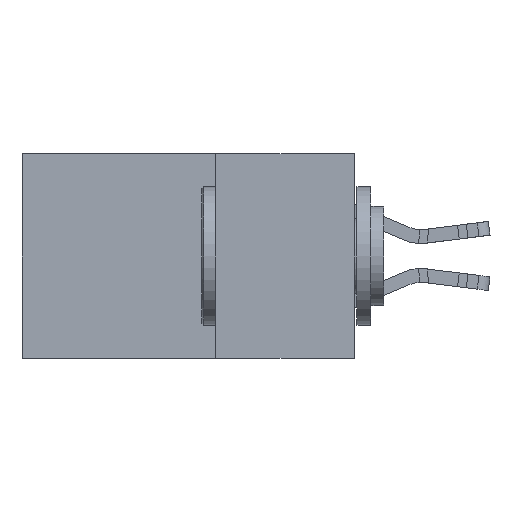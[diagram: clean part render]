
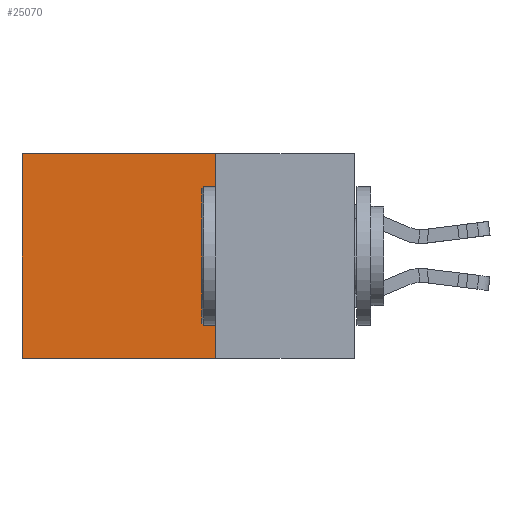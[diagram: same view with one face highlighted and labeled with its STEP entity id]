
A CAD part, left-side view. The second image highlights one B-rep face of the part: STEP entity #25070.
In plain terms, the highlighted planar face has unit normal (-1, 0, 0).
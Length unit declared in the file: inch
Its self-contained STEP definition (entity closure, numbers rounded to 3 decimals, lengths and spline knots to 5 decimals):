
#2036 = LINE ( 'NONE', #15305, #8247 ) ;
#2154 = VERTEX_POINT ( 'NONE', #5412 ) ;
#3725 = ORIENTED_EDGE ( 'NONE', *, *, #26143, .F. ) ;
#4687 = CARTESIAN_POINT ( 'NONE',  ( 0.2615, 0.25, 0. ) ) ;
#5412 = CARTESIAN_POINT ( 'NONE',  ( 0.2615, 0.6, 0. ) ) ;
#5791 = DIRECTION ( 'NONE',  ( 0., 1., 0. ) ) ;
#7809 = VECTOR ( 'NONE', #26336, 39.37008 ) ;
#8247 = VECTOR ( 'NONE', #10985, 39.37008 ) ;
#9611 = LINE ( 'NONE', #22758, #19324 ) ;
#10749 = VERTEX_POINT ( 'NONE', #24547 ) ;
#10985 = DIRECTION ( 'NONE',  ( 0., 0., -1. ) ) ;
#11311 = CARTESIAN_POINT ( 'NONE',  ( 0.2615, 0.25, -0.37 ) ) ;
#11790 = DIRECTION ( 'NONE',  ( 0., 1., 0. ) ) ;
#13046 = LINE ( 'NONE', #11311, #7809 ) ;
#13048 = VERTEX_POINT ( 'NONE', #4687 ) ;
#13764 = AXIS2_PLACEMENT_3D ( 'NONE', #16901, #25729, #23549 ) ;
#14367 = EDGE_LOOP ( 'NONE', ( #25754, #23099, #3725, #15654 ) ) ;
#14872 = LINE ( 'NONE', #25610, #21187 ) ;
#15262 = EDGE_CURVE ( 'NONE', #16244, #10749, #9611, .T. ) ;
#15305 = CARTESIAN_POINT ( 'NONE',  ( 0.2615, 0.6, -0.37 ) ) ;
#15654 = ORIENTED_EDGE ( 'NONE', *, *, #15926, .T. ) ;
#15926 = EDGE_CURVE ( 'NONE', #13048, #2154, #14872, .T. ) ;
#16244 = VERTEX_POINT ( 'NONE', #20388 ) ;
#16901 = CARTESIAN_POINT ( 'NONE',  ( 0.2615, 0.25, -0.37 ) ) ;
#17323 = EDGE_CURVE ( 'NONE', #2154, #10749, #2036, .T. ) ;
#18936 = FACE_OUTER_BOUND ( 'NONE', #14367, .T. ) ;
#19324 = VECTOR ( 'NONE', #11790, 39.37008 ) ;
#20388 = CARTESIAN_POINT ( 'NONE',  ( 0.2615, 0.25, -0.37 ) ) ;
#21187 = VECTOR ( 'NONE', #5791, 39.37008 ) ;
#22758 = CARTESIAN_POINT ( 'NONE',  ( 0.2615, 0.25, -0.37 ) ) ;
#23099 = ORIENTED_EDGE ( 'NONE', *, *, #15262, .F. ) ;
#23275 = PLANE ( 'NONE',  #13764 ) ;
#23549 = DIRECTION ( 'NONE',  ( 0., 0., -1. ) ) ;
#24547 = CARTESIAN_POINT ( 'NONE',  ( 0.2615, 0.6, -0.37 ) ) ;
#25070 = ADVANCED_FACE ( 'NONE', ( #18936 ), #23275, .F. ) ;
#25610 = CARTESIAN_POINT ( 'NONE',  ( 0.2615, 0.25, 0. ) ) ;
#25729 = DIRECTION ( 'NONE',  ( 1., 0., 0. ) ) ;
#25754 = ORIENTED_EDGE ( 'NONE', *, *, #17323, .T. ) ;
#26143 = EDGE_CURVE ( 'NONE', #13048, #16244, #13046, .T. ) ;
#26336 = DIRECTION ( 'NONE',  ( 0., 0., -1. ) ) ;
